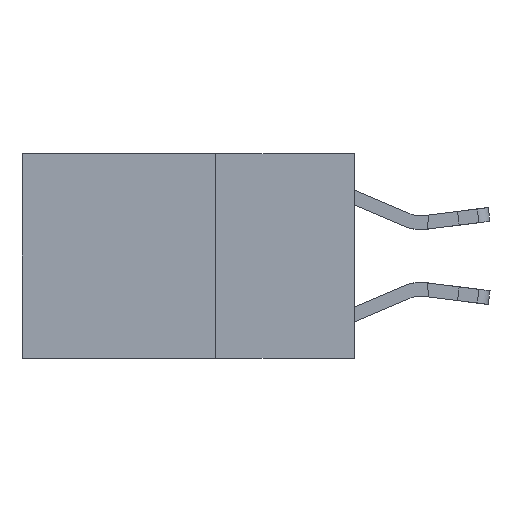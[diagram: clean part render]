
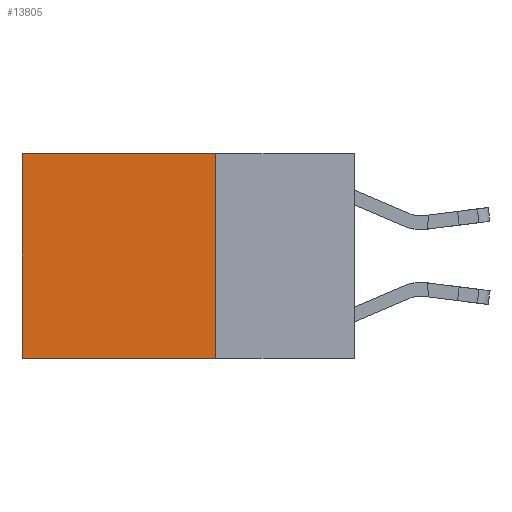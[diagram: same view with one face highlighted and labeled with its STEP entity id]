
A CAD part, left-side view. The second image highlights one B-rep face of the part: STEP entity #13805.
In plain terms, the highlighted planar face has unit normal (-1, 0, 0).
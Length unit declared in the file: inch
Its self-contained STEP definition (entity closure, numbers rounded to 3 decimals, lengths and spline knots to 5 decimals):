
#990 = LINE ( 'NONE', #1715, #12836 ) ;
#1212 = VECTOR ( 'NONE', #6365, 39.37008 ) ;
#1715 = CARTESIAN_POINT ( 'NONE',  ( 0.2625, 0.25, 0. ) ) ;
#1824 = VECTOR ( 'NONE', #11766, 39.37008 ) ;
#2554 = EDGE_CURVE ( 'NONE', #8281, #10536, #10994, .T. ) ;
#2593 = DIRECTION ( 'NONE',  ( 1., 0., 0. ) ) ;
#2729 = ORIENTED_EDGE ( 'NONE', *, *, #2554, .F. ) ;
#2737 = CARTESIAN_POINT ( 'NONE',  ( 0.2625, 0.25, 0. ) ) ;
#4256 = ORIENTED_EDGE ( 'NONE', *, *, #8381, .T. ) ;
#4656 = VECTOR ( 'NONE', #5408, 39.37008 ) ;
#5148 = ORIENTED_EDGE ( 'NONE', *, *, #12847, .F. ) ;
#5408 = DIRECTION ( 'NONE',  ( 0., 1., 0. ) ) ;
#6230 = EDGE_LOOP ( 'NONE', ( #8158, #5148, #2729, #4256 ) ) ;
#6320 = CARTESIAN_POINT ( 'NONE',  ( 0.2625, 0.6, -0.37 ) ) ;
#6365 = DIRECTION ( 'NONE',  ( 0., 0., -1. ) ) ;
#6487 = VERTEX_POINT ( 'NONE', #6320 ) ;
#6523 = EDGE_CURVE ( 'NONE', #11111, #6487, #8076, .T. ) ;
#8076 = LINE ( 'NONE', #13133, #1212 ) ;
#8158 = ORIENTED_EDGE ( 'NONE', *, *, #6523, .T. ) ;
#8281 = VERTEX_POINT ( 'NONE', #2737 ) ;
#8348 = PLANE ( 'NONE',  #8809 ) ;
#8381 = EDGE_CURVE ( 'NONE', #8281, #11111, #990, .T. ) ;
#8809 = AXIS2_PLACEMENT_3D ( 'NONE', #12845, #2593, #10638 ) ;
#9185 = CARTESIAN_POINT ( 'NONE',  ( 0.2625, 0.6, 0. ) ) ;
#10536 = VERTEX_POINT ( 'NONE', #12374 ) ;
#10638 = DIRECTION ( 'NONE',  ( 0., 0., -1. ) ) ;
#10994 = LINE ( 'NONE', #11821, #1824 ) ;
#11111 = VERTEX_POINT ( 'NONE', #9185 ) ;
#11766 = DIRECTION ( 'NONE',  ( 0., 0., -1. ) ) ;
#11821 = CARTESIAN_POINT ( 'NONE',  ( 0.2625, 0.25, 0. ) ) ;
#12065 = DIRECTION ( 'NONE',  ( 0., 1., 0. ) ) ;
#12198 = CARTESIAN_POINT ( 'NONE',  ( 0.2625, 0.25, -0.37 ) ) ;
#12374 = CARTESIAN_POINT ( 'NONE',  ( 0.2625, 0.25, -0.37 ) ) ;
#12836 = VECTOR ( 'NONE', #12065, 39.37008 ) ;
#12845 = CARTESIAN_POINT ( 'NONE',  ( 0.2625, 0.25, 0. ) ) ;
#12847 = EDGE_CURVE ( 'NONE', #10536, #6487, #13702, .T. ) ;
#12991 = FACE_OUTER_BOUND ( 'NONE', #6230, .T. ) ;
#13133 = CARTESIAN_POINT ( 'NONE',  ( 0.2625, 0.6, 0. ) ) ;
#13702 = LINE ( 'NONE', #12198, #4656 ) ;
#13805 = ADVANCED_FACE ( 'NONE', ( #12991 ), #8348, .F. ) ;
